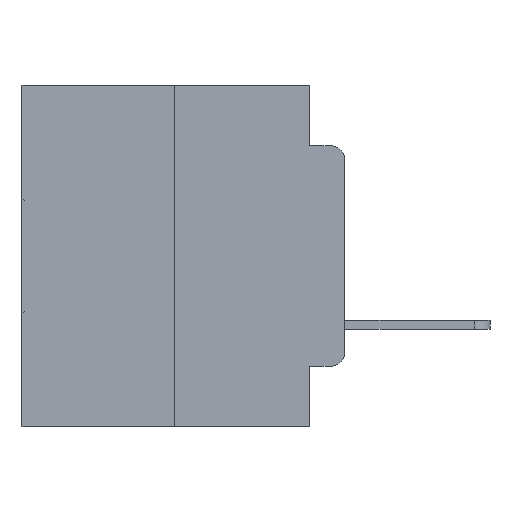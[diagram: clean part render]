
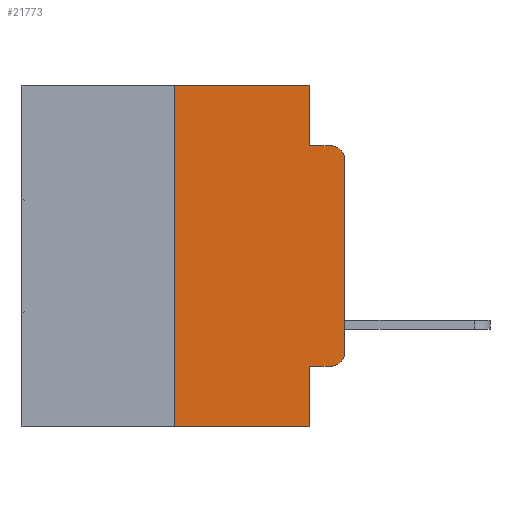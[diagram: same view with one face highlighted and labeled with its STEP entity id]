
A CAD part, left-side view. The second image highlights one B-rep face of the part: STEP entity #21773.
In plain terms, the highlighted planar face has unit normal (-1, 0, 0).
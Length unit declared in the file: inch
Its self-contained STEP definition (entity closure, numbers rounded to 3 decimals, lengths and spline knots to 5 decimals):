
#434 = VERTEX_POINT ( 'NONE', #18955 ) ;
#864 = CARTESIAN_POINT ( 'NONE',  ( 0., 0.25, -0.5 ) ) ;
#1949 = CARTESIAN_POINT ( 'NONE',  ( 0., 0.473, -0.5 ) ) ;
#2059 = CARTESIAN_POINT ( 'NONE',  ( 0., 0.473, 0. ) ) ;
#2725 = VERTEX_POINT ( 'NONE', #8131 ) ;
#2859 = VERTEX_POINT ( 'NONE', #22121 ) ;
#2952 = VECTOR ( 'NONE', #19010, 39.37008 ) ;
#3876 = EDGE_CURVE ( 'NONE', #27613, #17337, #20405, .T. ) ;
#4099 = CARTESIAN_POINT ( 'NONE',  ( 0., 0.051, 0. ) ) ;
#4604 = DIRECTION ( 'NONE',  ( 0., -1., 0. ) ) ;
#4734 = DIRECTION ( 'NONE',  ( 0., 0., -1. ) ) ;
#4757 = VERTEX_POINT ( 'NONE', #864 ) ;
#5110 = DIRECTION ( 'NONE',  ( 0., 0., -1. ) ) ;
#5227 = DIRECTION ( 'NONE',  ( -1., 0., 0. ) ) ;
#5357 = CIRCLE ( 'NONE', #6852, 0.02 ) ;
#5496 = CARTESIAN_POINT ( 'NONE',  ( 0., 0.02, -0.1085 ) ) ;
#5506 = LINE ( 'NONE', #22077, #18337 ) ;
#5762 = DIRECTION ( 'NONE',  ( 0., -1., 0. ) ) ;
#6053 = EDGE_LOOP ( 'NONE', ( #11112, #10627, #10158, #9776, #20453, #12778, #18359, #17928, #22059, #22658 ) ) ;
#6178 = EDGE_CURVE ( 'NONE', #434, #28897, #21923, .T. ) ;
#6799 = EDGE_CURVE ( 'NONE', #28897, #2859, #7799, .T. ) ;
#6852 = AXIS2_PLACEMENT_3D ( 'NONE', #10217, #25940, #12666 ) ;
#7142 = AXIS2_PLACEMENT_3D ( 'NONE', #2059, #19159, #4734 ) ;
#7214 = PLANE ( 'NONE',  #7142 ) ;
#7423 = EDGE_CURVE ( 'NONE', #28274, #2859, #17505, .T. ) ;
#7763 = LINE ( 'NONE', #4099, #12723 ) ;
#7799 = CIRCLE ( 'NONE', #22319, 0.02 ) ;
#8131 = CARTESIAN_POINT ( 'NONE',  ( 0., 0.25, 0. ) ) ;
#8565 = VECTOR ( 'NONE', #16782, 39.37008 ) ;
#8901 = VERTEX_POINT ( 'NONE', #16141 ) ;
#9776 = ORIENTED_EDGE ( 'NONE', *, *, #28709, .F. ) ;
#10158 = ORIENTED_EDGE ( 'NONE', *, *, #7423, .F. ) ;
#10217 = CARTESIAN_POINT ( 'NONE',  ( 0., 0.02, -0.3915 ) ) ;
#10627 = ORIENTED_EDGE ( 'NONE', *, *, #6799, .T. ) ;
#10780 = VERTEX_POINT ( 'NONE', #15056 ) ;
#11112 = ORIENTED_EDGE ( 'NONE', *, *, #6178, .T. ) ;
#11188 = LINE ( 'NONE', #14614, #17478 ) ;
#12370 = CARTESIAN_POINT ( 'NONE',  ( 0., 0.051, -0.4115 ) ) ;
#12562 = CARTESIAN_POINT ( 'NONE',  ( 0., 0., -0.1085 ) ) ;
#12666 = DIRECTION ( 'NONE',  ( 0., 0., -1. ) ) ;
#12723 = VECTOR ( 'NONE', #18659, 39.37008 ) ;
#12778 = ORIENTED_EDGE ( 'NONE', *, *, #24107, .F. ) ;
#14434 = CARTESIAN_POINT ( 'NONE',  ( 0., 0.051, 0. ) ) ;
#14614 = CARTESIAN_POINT ( 'NONE',  ( 0., 0.25, 0. ) ) ;
#14897 = EDGE_CURVE ( 'NONE', #2725, #10780, #5506, .T. ) ;
#14947 = LINE ( 'NONE', #1949, #25920 ) ;
#15056 = CARTESIAN_POINT ( 'NONE',  ( 0., 0.051, 0. ) ) ;
#15711 = DIRECTION ( 'NONE',  ( 0., -1., 0. ) ) ;
#15838 = CARTESIAN_POINT ( 'NONE',  ( 0., 0.051, -0.0885 ) ) ;
#16141 = CARTESIAN_POINT ( 'NONE',  ( 0., 0.051, -0.5 ) ) ;
#16172 = CARTESIAN_POINT ( 'NONE',  ( 0., 0.02, -0.4115 ) ) ;
#16782 = DIRECTION ( 'NONE',  ( 0., 0., -1. ) ) ;
#16989 = DIRECTION ( 'NONE',  ( 0., 0., 1. ) ) ;
#17337 = VERTEX_POINT ( 'NONE', #16172 ) ;
#17478 = VECTOR ( 'NONE', #16989, 39.37008 ) ;
#17505 = LINE ( 'NONE', #15838, #28203 ) ;
#17545 = CARTESIAN_POINT ( 'NONE',  ( 0., 0., 0. ) ) ;
#17550 = CARTESIAN_POINT ( 'NONE',  ( 0., 0.051, -0.4115 ) ) ;
#17630 = EDGE_CURVE ( 'NONE', #17337, #434, #5357, .T. ) ;
#17928 = ORIENTED_EDGE ( 'NONE', *, *, #29335, .F. ) ;
#18337 = VECTOR ( 'NONE', #5762, 39.37008 ) ;
#18359 = ORIENTED_EDGE ( 'NONE', *, *, #28710, .T. ) ;
#18659 = DIRECTION ( 'NONE',  ( 0., 0., -1. ) ) ;
#18955 = CARTESIAN_POINT ( 'NONE',  ( 0., 0., -0.3915 ) ) ;
#19010 = DIRECTION ( 'NONE',  ( 0., 0., 1. ) ) ;
#19159 = DIRECTION ( 'NONE',  ( 1., 0., 0. ) ) ;
#20405 = LINE ( 'NONE', #12370, #25399 ) ;
#20453 = ORIENTED_EDGE ( 'NONE', *, *, #14897, .F. ) ;
#21536 = LINE ( 'NONE', #14434, #8565 ) ;
#21773 = ADVANCED_FACE ( 'NONE', ( #22611 ), #7214, .F. ) ;
#21923 = LINE ( 'NONE', #17545, #2952 ) ;
#22059 = ORIENTED_EDGE ( 'NONE', *, *, #3876, .T. ) ;
#22077 = CARTESIAN_POINT ( 'NONE',  ( 0., 0.473, 0. ) ) ;
#22121 = CARTESIAN_POINT ( 'NONE',  ( 0., 0.02, -0.0885 ) ) ;
#22319 = AXIS2_PLACEMENT_3D ( 'NONE', #5496, #5227, #5110 ) ;
#22611 = FACE_OUTER_BOUND ( 'NONE', #6053, .T. ) ;
#22658 = ORIENTED_EDGE ( 'NONE', *, *, #17630, .T. ) ;
#24107 = EDGE_CURVE ( 'NONE', #4757, #2725, #11188, .T. ) ;
#24187 = CARTESIAN_POINT ( 'NONE',  ( 0., 0.051, -0.0885 ) ) ;
#25399 = VECTOR ( 'NONE', #27594, 39.37008 ) ;
#25920 = VECTOR ( 'NONE', #4604, 39.37008 ) ;
#25940 = DIRECTION ( 'NONE',  ( -1., 0., 0. ) ) ;
#27594 = DIRECTION ( 'NONE',  ( 0., -1., 0. ) ) ;
#27613 = VERTEX_POINT ( 'NONE', #17550 ) ;
#28203 = VECTOR ( 'NONE', #15711, 39.37008 ) ;
#28274 = VERTEX_POINT ( 'NONE', #24187 ) ;
#28709 = EDGE_CURVE ( 'NONE', #10780, #28274, #21536, .T. ) ;
#28710 = EDGE_CURVE ( 'NONE', #4757, #8901, #14947, .T. ) ;
#28897 = VERTEX_POINT ( 'NONE', #12562 ) ;
#29335 = EDGE_CURVE ( 'NONE', #27613, #8901, #7763, .T. ) ;
